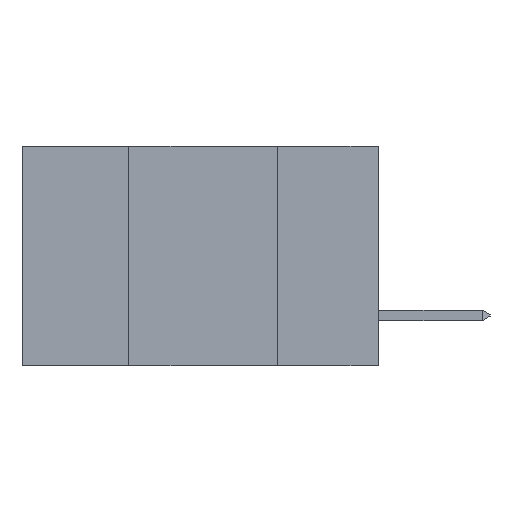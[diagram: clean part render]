
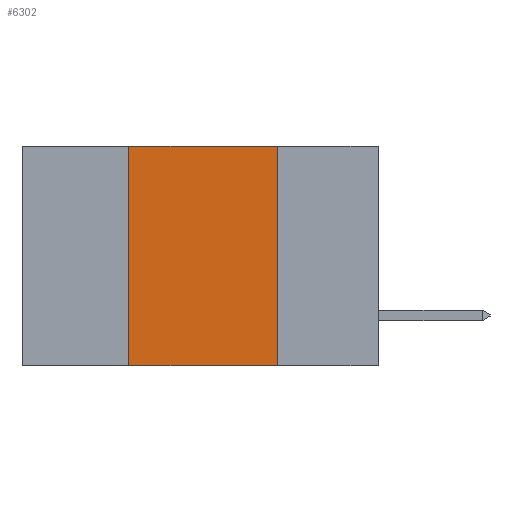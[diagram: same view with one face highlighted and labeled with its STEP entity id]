
A CAD part, left-side view. The second image highlights one B-rep face of the part: STEP entity #6302.
In plain terms, the highlighted planar face has unit normal (-1, 0, 0).
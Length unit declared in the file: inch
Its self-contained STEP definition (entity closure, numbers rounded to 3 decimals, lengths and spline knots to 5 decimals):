
#6 = CARTESIAN_POINT ( 'NONE',  ( 0., 0.6, 0. ) ) ;
#104 = CARTESIAN_POINT ( 'NONE',  ( 0., 0.42, 0. ) ) ;
#1051 = LINE ( 'NONE', #8498, #6596 ) ;
#1112 = CARTESIAN_POINT ( 'NONE',  ( 0., 0.42, -0.37 ) ) ;
#1195 = DIRECTION ( 'NONE',  ( 0., -1., 0. ) ) ;
#1585 = VERTEX_POINT ( 'NONE', #6994 ) ;
#1588 = ORIENTED_EDGE ( 'NONE', *, *, #8802, .F. ) ;
#1623 = VERTEX_POINT ( 'NONE', #5842 ) ;
#1779 = EDGE_LOOP ( 'NONE', ( #6769, #12502, #1588, #10153 ) ) ;
#2192 = VECTOR ( 'NONE', #11240, 39.37008 ) ;
#2317 = FACE_OUTER_BOUND ( 'NONE', #1779, .T. ) ;
#2624 = DIRECTION ( 'NONE',  ( 1., 0., 0. ) ) ;
#2644 = DIRECTION ( 'NONE',  ( 0., 0., -1. ) ) ;
#2753 = PLANE ( 'NONE',  #8976 ) ;
#3895 = LINE ( 'NONE', #6292, #11847 ) ;
#4175 = VERTEX_POINT ( 'NONE', #104 ) ;
#5303 = EDGE_CURVE ( 'NONE', #1623, #1585, #13005, .T. ) ;
#5842 = CARTESIAN_POINT ( 'NONE',  ( 0., 0.17, 0. ) ) ;
#6292 = CARTESIAN_POINT ( 'NONE',  ( 0., 0.42, 0. ) ) ;
#6302 = ADVANCED_FACE ( 'NONE', ( #2317 ), #2753, .F. ) ;
#6596 = VECTOR ( 'NONE', #9527, 39.37008 ) ;
#6769 = ORIENTED_EDGE ( 'NONE', *, *, #5303, .F. ) ;
#6887 = LINE ( 'NONE', #6, #9302 ) ;
#6994 = CARTESIAN_POINT ( 'NONE',  ( 0., 0.17, -0.37 ) ) ;
#8498 = CARTESIAN_POINT ( 'NONE',  ( 0., 0.6, -0.37 ) ) ;
#8802 = EDGE_CURVE ( 'NONE', #13544, #4175, #3895, .T. ) ;
#8976 = AXIS2_PLACEMENT_3D ( 'NONE', #9856, #2624, #2644 ) ;
#9076 = EDGE_CURVE ( 'NONE', #4175, #1623, #6887, .T. ) ;
#9302 = VECTOR ( 'NONE', #1195, 39.37008 ) ;
#9426 = DIRECTION ( 'NONE',  ( 0., 0., 1. ) ) ;
#9527 = DIRECTION ( 'NONE',  ( 0., -1., 0. ) ) ;
#9856 = CARTESIAN_POINT ( 'NONE',  ( 0., 0.6, 0. ) ) ;
#10153 = ORIENTED_EDGE ( 'NONE', *, *, #10749, .T. ) ;
#10749 = EDGE_CURVE ( 'NONE', #13544, #1585, #1051, .T. ) ;
#11049 = CARTESIAN_POINT ( 'NONE',  ( 0., 0.17, 0. ) ) ;
#11240 = DIRECTION ( 'NONE',  ( 0., 0., -1. ) ) ;
#11847 = VECTOR ( 'NONE', #9426, 39.37008 ) ;
#12502 = ORIENTED_EDGE ( 'NONE', *, *, #9076, .F. ) ;
#13005 = LINE ( 'NONE', #11049, #2192 ) ;
#13544 = VERTEX_POINT ( 'NONE', #1112 ) ;
